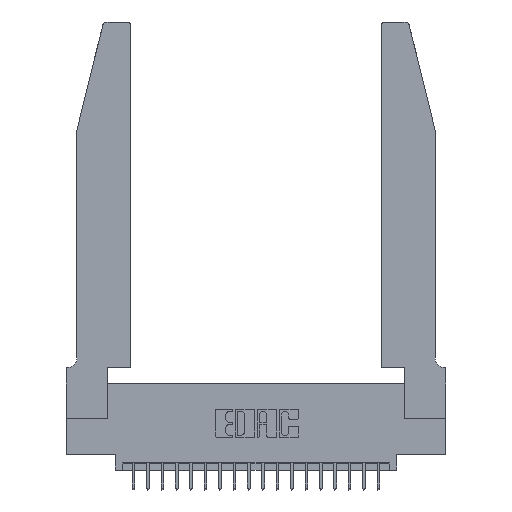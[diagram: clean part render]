
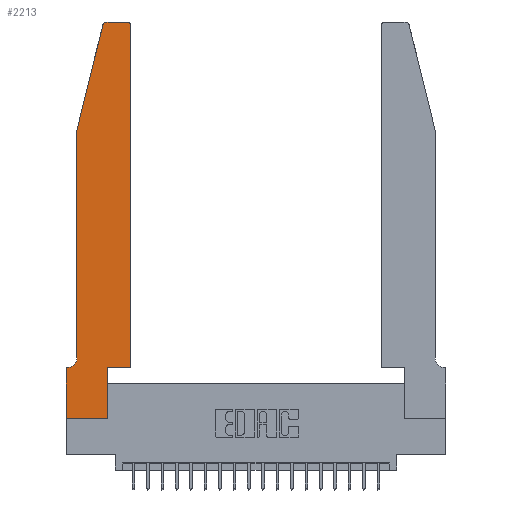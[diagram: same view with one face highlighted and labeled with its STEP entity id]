
A CAD part, top view. The second image highlights one B-rep face of the part: STEP entity #2213.
In plain terms, the highlighted planar face has unit normal (0, 0, 1).
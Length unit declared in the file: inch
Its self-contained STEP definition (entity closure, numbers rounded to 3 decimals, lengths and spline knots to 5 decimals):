
#46 = LINE ( 'NONE', #1741, #7653 ) ;
#405 = PLANE ( 'NONE',  #5432 ) ;
#417 = CARTESIAN_POINT ( 'NONE',  ( 0.4505, 2.72, 0.37 ) ) ;
#840 = CARTESIAN_POINT ( 'NONE',  ( 0.25487, 2.72718, 0.37 ) ) ;
#934 = CARTESIAN_POINT ( 'NONE',  ( 0.2605, 2.75, 0.37 ) ) ;
#1071 = ORIENTED_EDGE ( 'NONE', *, *, #8708, .T. ) ;
#1244 = LINE ( 'NONE', #2953, #13794 ) ;
#1741 = CARTESIAN_POINT ( 'NONE',  ( 0.4505, 0.35, 0.37 ) ) ;
#1784 = CARTESIAN_POINT ( 'NONE',  ( 0.2865, 0.35, 0.37 ) ) ;
#2213 = ADVANCED_FACE ( 'NONE', ( #10791 ), #405, .T. ) ;
#2722 = CARTESIAN_POINT ( 'NONE',  ( 0.0755, 2., 0.37 ) ) ;
#2763 = CARTESIAN_POINT ( 'NONE',  ( 0.0755, 0.42, 0.37 ) ) ;
#2953 = CARTESIAN_POINT ( 'NONE',  ( 0.4505, 0.35, 0.37 ) ) ;
#3183 = DIRECTION ( 'NONE',  ( 0., 1., 0. ) ) ;
#3221 = ORIENTED_EDGE ( 'NONE', *, *, #17942, .T. ) ;
#3223 = CARTESIAN_POINT ( 'NONE',  ( 0.4205, 2.75, 0.37 ) ) ;
#3304 = DIRECTION ( 'NONE',  ( 0., -1., 0. ) ) ;
#3421 = CARTESIAN_POINT ( 'NONE',  ( 0., 0., 0.37 ) ) ;
#3442 = CARTESIAN_POINT ( 'NONE',  ( 0.2865, 0., 0.37 ) ) ;
#3507 = CARTESIAN_POINT ( 'NONE',  ( 0.4505, 0.35, 0.37 ) ) ;
#3748 = ORIENTED_EDGE ( 'NONE', *, *, #17889, .T. ) ;
#3942 = EDGE_LOOP ( 'NONE', ( #4642, #3221, #18240, #3748, #7990, #8692, #17927, #18897, #9666, #12240, #21772, #1071 ) ) ;
#4642 = ORIENTED_EDGE ( 'NONE', *, *, #12521, .T. ) ;
#4815 = DIRECTION ( 'NONE',  ( -1., 0., 0. ) ) ;
#5176 = VERTEX_POINT ( 'NONE', #7853 ) ;
#5293 = VECTOR ( 'NONE', #13057, 39.37008 ) ;
#5409 = DIRECTION ( 'NONE',  ( 1., 0., 0. ) ) ;
#5432 = AXIS2_PLACEMENT_3D ( 'NONE', #7407, #15649, #7079 ) ;
#5497 = CARTESIAN_POINT ( 'NONE',  ( 0.0055, 0.42, 0.37 ) ) ;
#5791 = VECTOR ( 'NONE', #17142, 39.37008 ) ;
#6243 = DIRECTION ( 'NONE',  ( 1., 0., 0. ) ) ;
#6332 = CARTESIAN_POINT ( 'NONE',  ( 0., 0.35, 0.37 ) ) ;
#6469 = LINE ( 'NONE', #934, #10667 ) ;
#6804 = VERTEX_POINT ( 'NONE', #3442 ) ;
#7079 = DIRECTION ( 'NONE',  ( 1., 0., 0. ) ) ;
#7198 = DIRECTION ( 'NONE',  ( 0., 0., 1. ) ) ;
#7407 = CARTESIAN_POINT ( 'NONE',  ( 0., 0.35, 0.37 ) ) ;
#7518 = LINE ( 'NONE', #21962, #5791 ) ;
#7528 = VECTOR ( 'NONE', #18625, 39.37008 ) ;
#7580 = AXIS2_PLACEMENT_3D ( 'NONE', #10918, #7198, #5409 ) ;
#7653 = VECTOR ( 'NONE', #12042, 39.37008 ) ;
#7853 = CARTESIAN_POINT ( 'NONE',  ( 0., 0., 0.37 ) ) ;
#7990 = ORIENTED_EDGE ( 'NONE', *, *, #8343, .T. ) ;
#8343 = EDGE_CURVE ( 'NONE', #11648, #9543, #17076, .T. ) ;
#8363 = EDGE_CURVE ( 'NONE', #20523, #14673, #46, .T. ) ;
#8371 = DIRECTION ( 'NONE',  ( -0.239, -0.971, 0. ) ) ;
#8692 = ORIENTED_EDGE ( 'NONE', *, *, #18041, .T. ) ;
#8708 = EDGE_CURVE ( 'NONE', #21894, #12054, #11205, .T. ) ;
#8718 = VECTOR ( 'NONE', #3304, 39.37008 ) ;
#8755 = AXIS2_PLACEMENT_3D ( 'NONE', #5497, #17148, #12153 ) ;
#9352 = CIRCLE ( 'NONE', #7580, 0.03 ) ;
#9543 = VERTEX_POINT ( 'NONE', #12366 ) ;
#9666 = ORIENTED_EDGE ( 'NONE', *, *, #12381, .T. ) ;
#9714 = CARTESIAN_POINT ( 'NONE',  ( 0., 0., 0.37 ) ) ;
#10113 = VERTEX_POINT ( 'NONE', #17058 ) ;
#10388 = CARTESIAN_POINT ( 'NONE',  ( 0.0755, 2., 0.37 ) ) ;
#10667 = VECTOR ( 'NONE', #4815, 39.37008 ) ;
#10791 = FACE_OUTER_BOUND ( 'NONE', #3942, .T. ) ;
#10918 = CARTESIAN_POINT ( 'NONE',  ( 0.284, 2.72, 0.37 ) ) ;
#11205 = CIRCLE ( 'NONE', #14114, 0.03 ) ;
#11238 = LINE ( 'NONE', #11836, #7528 ) ;
#11648 = VERTEX_POINT ( 'NONE', #2763 ) ;
#11836 = CARTESIAN_POINT ( 'NONE',  ( 0.0755, 2., 0.37 ) ) ;
#12042 = DIRECTION ( 'NONE',  ( 1., 0., 0. ) ) ;
#12054 = VERTEX_POINT ( 'NONE', #3223 ) ;
#12153 = DIRECTION ( 'NONE',  ( -1., 0., 0. ) ) ;
#12240 = ORIENTED_EDGE ( 'NONE', *, *, #8363, .T. ) ;
#12366 = CARTESIAN_POINT ( 'NONE',  ( 0.0055, 0.35, 0.37 ) ) ;
#12381 = EDGE_CURVE ( 'NONE', #6804, #20523, #15173, .T. ) ;
#12521 = EDGE_CURVE ( 'NONE', #12054, #10113, #6469, .T. ) ;
#12815 = VERTEX_POINT ( 'NONE', #2722 ) ;
#12900 = VERTEX_POINT ( 'NONE', #6332 ) ;
#13057 = DIRECTION ( 'NONE',  ( 0., 1., 0. ) ) ;
#13380 = CARTESIAN_POINT ( 'NONE',  ( 0.4205, 2.72, 0.37 ) ) ;
#13794 = VECTOR ( 'NONE', #3183, 39.37008 ) ;
#14114 = AXIS2_PLACEMENT_3D ( 'NONE', #13380, #18575, #6243 ) ;
#14673 = VERTEX_POINT ( 'NONE', #3507 ) ;
#15173 = LINE ( 'NONE', #21945, #5293 ) ;
#15481 = LINE ( 'NONE', #10388, #20592 ) ;
#15649 = DIRECTION ( 'NONE',  ( 0., 0., 1. ) ) ;
#16585 = VECTOR ( 'NONE', #20234, 39.37008 ) ;
#17058 = CARTESIAN_POINT ( 'NONE',  ( 0.284, 2.75, 0.37 ) ) ;
#17076 = CIRCLE ( 'NONE', #8755, 0.07 ) ;
#17142 = DIRECTION ( 'NONE',  ( -1., 0., 0. ) ) ;
#17148 = DIRECTION ( 'NONE',  ( 0., 0., -1. ) ) ;
#17818 = VERTEX_POINT ( 'NONE', #840 ) ;
#17889 = EDGE_CURVE ( 'NONE', #12815, #11648, #11238, .T. ) ;
#17927 = ORIENTED_EDGE ( 'NONE', *, *, #21971, .T. ) ;
#17942 = EDGE_CURVE ( 'NONE', #10113, #17818, #9352, .T. ) ;
#18041 = EDGE_CURVE ( 'NONE', #9543, #12900, #7518, .T. ) ;
#18240 = ORIENTED_EDGE ( 'NONE', *, *, #20021, .T. ) ;
#18575 = DIRECTION ( 'NONE',  ( 0., 0., 1. ) ) ;
#18625 = DIRECTION ( 'NONE',  ( 0., -1., 0. ) ) ;
#18802 = LINE ( 'NONE', #3421, #8718 ) ;
#18897 = ORIENTED_EDGE ( 'NONE', *, *, #19452, .T. ) ;
#19452 = EDGE_CURVE ( 'NONE', #5176, #6804, #22032, .T. ) ;
#20021 = EDGE_CURVE ( 'NONE', #17818, #12815, #15481, .T. ) ;
#20234 = DIRECTION ( 'NONE',  ( 1., 0., 0. ) ) ;
#20523 = VERTEX_POINT ( 'NONE', #1784 ) ;
#20592 = VECTOR ( 'NONE', #8371, 39.37008 ) ;
#21772 = ORIENTED_EDGE ( 'NONE', *, *, #21982, .T. ) ;
#21894 = VERTEX_POINT ( 'NONE', #417 ) ;
#21945 = CARTESIAN_POINT ( 'NONE',  ( 0.2865, 0.35, 0.37 ) ) ;
#21962 = CARTESIAN_POINT ( 'NONE',  ( 0.0755, 0.35, 0.37 ) ) ;
#21971 = EDGE_CURVE ( 'NONE', #12900, #5176, #18802, .T. ) ;
#21982 = EDGE_CURVE ( 'NONE', #14673, #21894, #1244, .T. ) ;
#22032 = LINE ( 'NONE', #9714, #16585 ) ;
